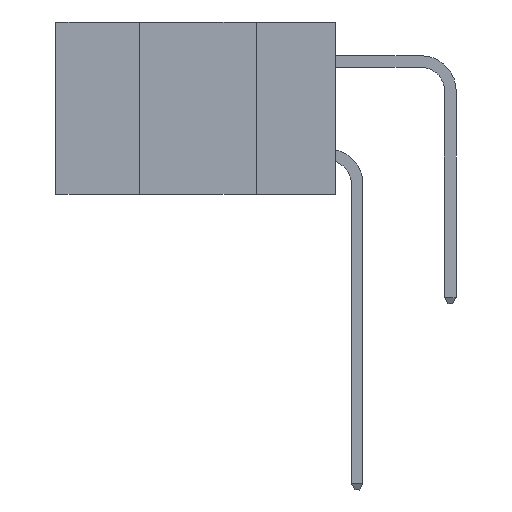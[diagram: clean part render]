
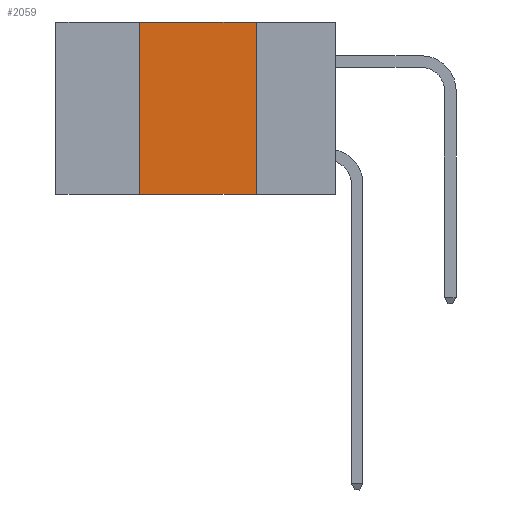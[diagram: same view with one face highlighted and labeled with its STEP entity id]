
A CAD part, left-side view. The second image highlights one B-rep face of the part: STEP entity #2059.
In plain terms, the highlighted planar face has unit normal (-1, 0, 0).
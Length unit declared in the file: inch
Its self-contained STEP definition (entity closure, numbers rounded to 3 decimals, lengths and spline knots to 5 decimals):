
#57 = VERTEX_POINT ( 'NONE', #82 ) ;
#82 = CARTESIAN_POINT ( 'NONE',  ( 0., 0.42, -0.37 ) ) ;
#284 = EDGE_CURVE ( 'NONE', #9416, #7745, #3281, .T. ) ;
#316 = CARTESIAN_POINT ( 'NONE',  ( 0., 0.17, -0.37 ) ) ;
#958 = LINE ( 'NONE', #4531, #10014 ) ;
#1000 = VERTEX_POINT ( 'NONE', #4751 ) ;
#1043 = VECTOR ( 'NONE', #5637, 39.37008 ) ;
#1290 = CARTESIAN_POINT ( 'NONE',  ( 0., 0.17, 0. ) ) ;
#1613 = ORIENTED_EDGE ( 'NONE', *, *, #9126, .F. ) ;
#1785 = FACE_OUTER_BOUND ( 'NONE', #7360, .T. ) ;
#1806 = ORIENTED_EDGE ( 'NONE', *, *, #2512, .F. ) ;
#1908 = PLANE ( 'NONE',  #11107 ) ;
#2059 = ADVANCED_FACE ( 'NONE', ( #1785 ), #1908, .F. ) ;
#2512 = EDGE_CURVE ( 'NONE', #1000, #9416, #8341, .T. ) ;
#2674 = DIRECTION ( 'NONE',  ( 1., 0., 0. ) ) ;
#2728 = DIRECTION ( 'NONE',  ( 0., 0., -1. ) ) ;
#3281 = LINE ( 'NONE', #10484, #7819 ) ;
#3782 = CARTESIAN_POINT ( 'NONE',  ( 0., 0.6, -0.37 ) ) ;
#4531 = CARTESIAN_POINT ( 'NONE',  ( 0., 0.42, 0. ) ) ;
#4678 = LINE ( 'NONE', #3782, #6417 ) ;
#4751 = CARTESIAN_POINT ( 'NONE',  ( 0., 0.42, 0. ) ) ;
#5637 = DIRECTION ( 'NONE',  ( 0., -1., 0. ) ) ;
#6417 = VECTOR ( 'NONE', #10814, 39.37008 ) ;
#7360 = EDGE_LOOP ( 'NONE', ( #10409, #1806, #1613, #11457 ) ) ;
#7541 = CARTESIAN_POINT ( 'NONE',  ( 0., 0.6, 0. ) ) ;
#7745 = VERTEX_POINT ( 'NONE', #316 ) ;
#7819 = VECTOR ( 'NONE', #10666, 39.37008 ) ;
#8341 = LINE ( 'NONE', #7541, #1043 ) ;
#9126 = EDGE_CURVE ( 'NONE', #57, #1000, #958, .T. ) ;
#9416 = VERTEX_POINT ( 'NONE', #1290 ) ;
#9605 = EDGE_CURVE ( 'NONE', #57, #7745, #4678, .T. ) ;
#10014 = VECTOR ( 'NONE', #11744, 39.37008 ) ;
#10409 = ORIENTED_EDGE ( 'NONE', *, *, #284, .F. ) ;
#10484 = CARTESIAN_POINT ( 'NONE',  ( 0., 0.17, 0. ) ) ;
#10666 = DIRECTION ( 'NONE',  ( 0., 0., -1. ) ) ;
#10814 = DIRECTION ( 'NONE',  ( 0., -1., 0. ) ) ;
#10838 = CARTESIAN_POINT ( 'NONE',  ( 0., 0.6, 0. ) ) ;
#11107 = AXIS2_PLACEMENT_3D ( 'NONE', #10838, #2674, #2728 ) ;
#11457 = ORIENTED_EDGE ( 'NONE', *, *, #9605, .T. ) ;
#11744 = DIRECTION ( 'NONE',  ( 0., 0., 1. ) ) ;
